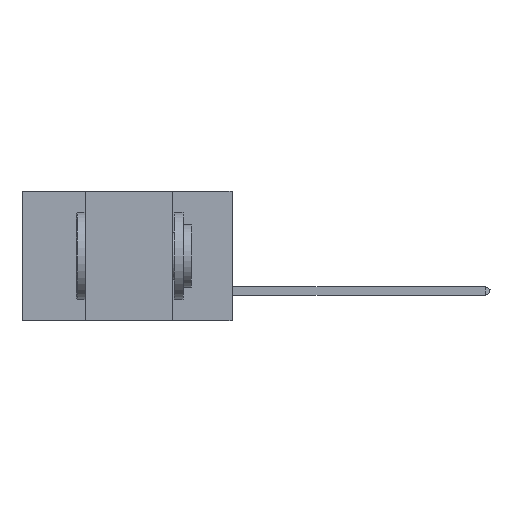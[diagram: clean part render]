
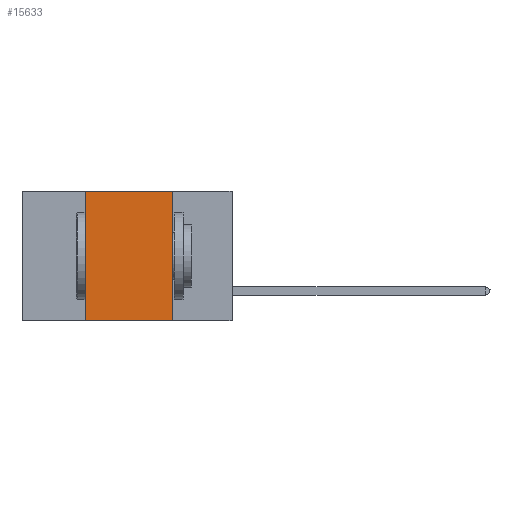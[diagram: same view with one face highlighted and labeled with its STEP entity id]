
A CAD part, left-side view. The second image highlights one B-rep face of the part: STEP entity #15633.
In plain terms, the highlighted planar face has unit normal (-1, 0, 0).
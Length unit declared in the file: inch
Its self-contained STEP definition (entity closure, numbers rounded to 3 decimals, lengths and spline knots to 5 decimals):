
#2623 = DIRECTION ( 'NONE',  ( 0., 0., 1. ) ) ;
#3101 = VECTOR ( 'NONE', #2623, 39.37008 ) ;
#3117 = VERTEX_POINT ( 'NONE', #19815 ) ;
#3542 = EDGE_CURVE ( 'NONE', #23110, #24007, #34755, .T. ) ;
#5380 = DIRECTION ( 'NONE',  ( 0., -1., 0. ) ) ;
#5400 = CARTESIAN_POINT ( 'NONE',  ( 0., 0.17, -0.37 ) ) ;
#7104 = FACE_OUTER_BOUND ( 'NONE', #28000, .T. ) ;
#9130 = AXIS2_PLACEMENT_3D ( 'NONE', #24744, #10028, #30764 ) ;
#9991 = DIRECTION ( 'NONE',  ( 0., 0., -1. ) ) ;
#10028 = DIRECTION ( 'NONE',  ( 1., 0., 0. ) ) ;
#11066 = ORIENTED_EDGE ( 'NONE', *, *, #16121, .F. ) ;
#12586 = ORIENTED_EDGE ( 'NONE', *, *, #3542, .F. ) ;
#14521 = VERTEX_POINT ( 'NONE', #5400 ) ;
#15114 = EDGE_CURVE ( 'NONE', #24007, #3117, #20548, .T. ) ;
#15633 = ADVANCED_FACE ( 'NONE', ( #7104 ), #15964, .F. ) ;
#15964 = PLANE ( 'NONE',  #9130 ) ;
#16121 = EDGE_CURVE ( 'NONE', #3117, #14521, #22985, .T. ) ;
#19495 = CARTESIAN_POINT ( 'NONE',  ( 0., 0.42, 0. ) ) ;
#19815 = CARTESIAN_POINT ( 'NONE',  ( 0., 0.17, 0. ) ) ;
#19876 = DIRECTION ( 'NONE',  ( 0., -1., 0. ) ) ;
#19902 = CARTESIAN_POINT ( 'NONE',  ( 0., 0.6, -0.37 ) ) ;
#20419 = CARTESIAN_POINT ( 'NONE',  ( 0., 0.42, 0. ) ) ;
#20548 = LINE ( 'NONE', #34859, #33126 ) ;
#21572 = VECTOR ( 'NONE', #5380, 39.37008 ) ;
#21893 = EDGE_CURVE ( 'NONE', #23110, #14521, #37013, .T. ) ;
#22985 = LINE ( 'NONE', #27734, #32783 ) ;
#23110 = VERTEX_POINT ( 'NONE', #33363 ) ;
#24007 = VERTEX_POINT ( 'NONE', #19495 ) ;
#24744 = CARTESIAN_POINT ( 'NONE',  ( 0., 0.6, 0. ) ) ;
#27734 = CARTESIAN_POINT ( 'NONE',  ( 0., 0.17, 0. ) ) ;
#28000 = EDGE_LOOP ( 'NONE', ( #11066, #31917, #12586, #31464 ) ) ;
#30764 = DIRECTION ( 'NONE',  ( 0., 0., -1. ) ) ;
#31464 = ORIENTED_EDGE ( 'NONE', *, *, #21893, .T. ) ;
#31917 = ORIENTED_EDGE ( 'NONE', *, *, #15114, .F. ) ;
#32783 = VECTOR ( 'NONE', #9991, 39.37008 ) ;
#33126 = VECTOR ( 'NONE', #19876, 39.37008 ) ;
#33363 = CARTESIAN_POINT ( 'NONE',  ( 0., 0.42, -0.37 ) ) ;
#34755 = LINE ( 'NONE', #20419, #3101 ) ;
#34859 = CARTESIAN_POINT ( 'NONE',  ( 0., 0.6, 0. ) ) ;
#37013 = LINE ( 'NONE', #19902, #21572 ) ;
